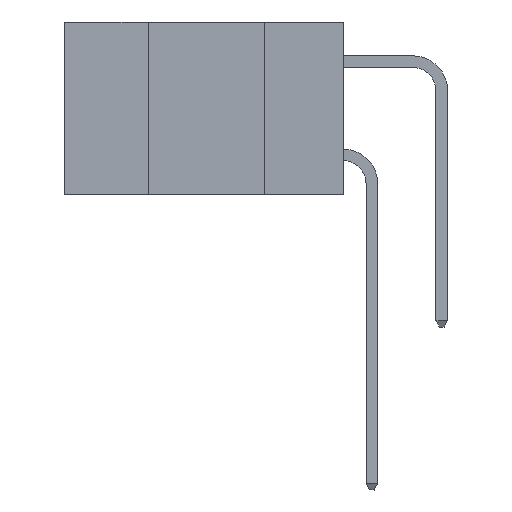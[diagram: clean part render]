
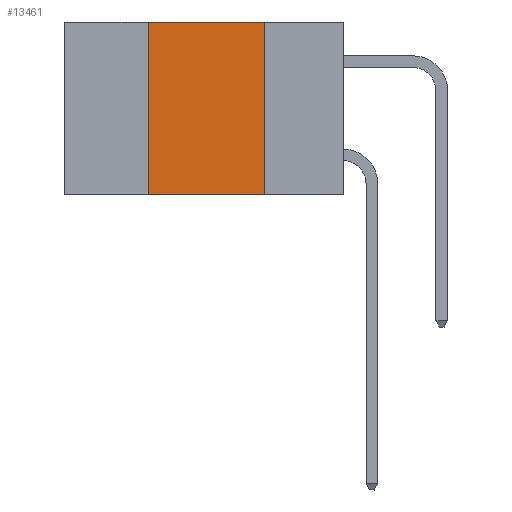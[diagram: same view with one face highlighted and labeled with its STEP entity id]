
A CAD part, left-side view. The second image highlights one B-rep face of the part: STEP entity #13461.
In plain terms, the highlighted planar face has unit normal (-1, 0, 0).
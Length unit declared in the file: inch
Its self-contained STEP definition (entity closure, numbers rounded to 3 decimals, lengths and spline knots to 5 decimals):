
#137 = DIRECTION ( 'NONE',  ( 0., 0., 1. ) ) ;
#242 = VERTEX_POINT ( 'NONE', #1205 ) ;
#429 = PLANE ( 'NONE',  #6176 ) ;
#1205 = CARTESIAN_POINT ( 'NONE',  ( 0., 0.42, 0. ) ) ;
#1247 = EDGE_CURVE ( 'NONE', #242, #9048, #7905, .T. ) ;
#1453 = LINE ( 'NONE', #5694, #13569 ) ;
#1535 = CARTESIAN_POINT ( 'NONE',  ( 0., 0.17, -0.37 ) ) ;
#2298 = LINE ( 'NONE', #4434, #10242 ) ;
#2471 = CARTESIAN_POINT ( 'NONE',  ( 0., 0.42, -0.37 ) ) ;
#3150 = VERTEX_POINT ( 'NONE', #1535 ) ;
#3428 = CARTESIAN_POINT ( 'NONE',  ( 0., 0.6, 0. ) ) ;
#3603 = DIRECTION ( 'NONE',  ( 0., -1., 0. ) ) ;
#4434 = CARTESIAN_POINT ( 'NONE',  ( 0., 0.42, -0.37 ) ) ;
#4661 = DIRECTION ( 'NONE',  ( 0., 0., -1. ) ) ;
#5032 = EDGE_LOOP ( 'NONE', ( #8197, #13407, #11477, #12999 ) ) ;
#5694 = CARTESIAN_POINT ( 'NONE',  ( 0., 0.17, -0.37 ) ) ;
#6176 = AXIS2_PLACEMENT_3D ( 'NONE', #3428, #8779, #4661 ) ;
#6179 = VECTOR ( 'NONE', #3603, 39.37008 ) ;
#6487 = EDGE_CURVE ( 'NONE', #9048, #3150, #1453, .T. ) ;
#7807 = FACE_OUTER_BOUND ( 'NONE', #5032, .T. ) ;
#7905 = LINE ( 'NONE', #13093, #6179 ) ;
#8031 = EDGE_CURVE ( 'NONE', #13007, #3150, #11454, .T. ) ;
#8197 = ORIENTED_EDGE ( 'NONE', *, *, #6487, .F. ) ;
#8779 = DIRECTION ( 'NONE',  ( 1., 0., 0. ) ) ;
#9034 = CARTESIAN_POINT ( 'NONE',  ( 0., 0.6, -0.37 ) ) ;
#9048 = VERTEX_POINT ( 'NONE', #13570 ) ;
#9563 = EDGE_CURVE ( 'NONE', #13007, #242, #2298, .T. ) ;
#9927 = DIRECTION ( 'NONE',  ( 0., 0., -1. ) ) ;
#10242 = VECTOR ( 'NONE', #137, 39.37008 ) ;
#11454 = LINE ( 'NONE', #9034, #12644 ) ;
#11477 = ORIENTED_EDGE ( 'NONE', *, *, #9563, .F. ) ;
#12644 = VECTOR ( 'NONE', #13246, 39.37008 ) ;
#12999 = ORIENTED_EDGE ( 'NONE', *, *, #8031, .T. ) ;
#13007 = VERTEX_POINT ( 'NONE', #2471 ) ;
#13093 = CARTESIAN_POINT ( 'NONE',  ( 0., 0.6, 0. ) ) ;
#13246 = DIRECTION ( 'NONE',  ( 0., -1., 0. ) ) ;
#13407 = ORIENTED_EDGE ( 'NONE', *, *, #1247, .F. ) ;
#13461 = ADVANCED_FACE ( 'NONE', ( #7807 ), #429, .F. ) ;
#13569 = VECTOR ( 'NONE', #9927, 39.37008 ) ;
#13570 = CARTESIAN_POINT ( 'NONE',  ( 0., 0.17, 0. ) ) ;
